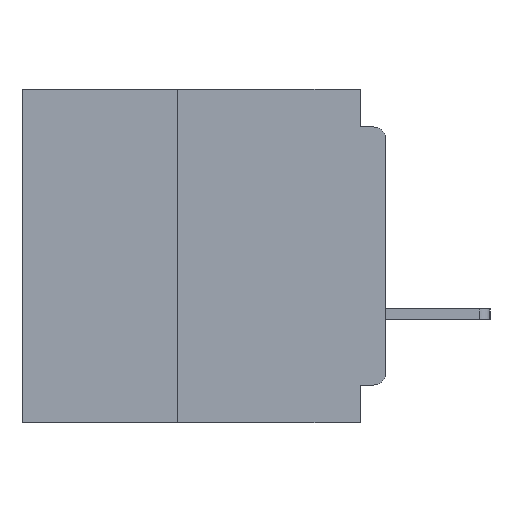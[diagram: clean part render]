
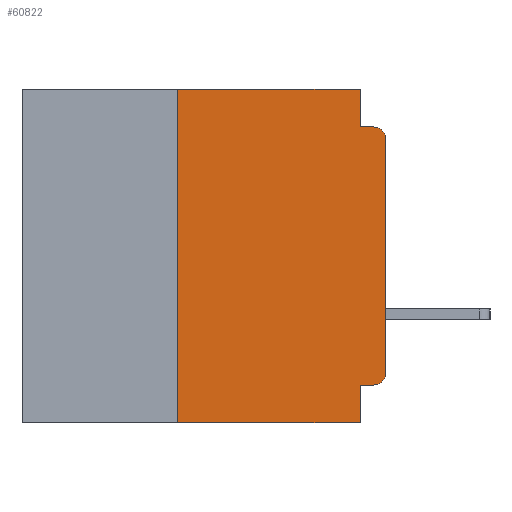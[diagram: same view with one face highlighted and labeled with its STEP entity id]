
A CAD part, left-side view. The second image highlights one B-rep face of the part: STEP entity #60822.
In plain terms, the highlighted planar face has unit normal (-1, 0, 0).
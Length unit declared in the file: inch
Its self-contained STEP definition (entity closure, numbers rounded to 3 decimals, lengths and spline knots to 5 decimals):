
#879 = VECTOR ( 'NONE', #21211, 39.37008 ) ;
#1084 = LINE ( 'NONE', #3844, #49012 ) ;
#2308 = LINE ( 'NONE', #2730, #51685 ) ;
#2730 = CARTESIAN_POINT ( 'NONE',  ( 0., 0.437, 0. ) ) ;
#3196 = LINE ( 'NONE', #24587, #39939 ) ;
#3844 = CARTESIAN_POINT ( 'NONE',  ( 0., 0.031, -0.4 ) ) ;
#6671 = LINE ( 'NONE', #43525, #29167 ) ;
#6939 = CARTESIAN_POINT ( 'NONE',  ( 0., 0.25, 0. ) ) ;
#6957 = AXIS2_PLACEMENT_3D ( 'NONE', #60217, #41269, #12670 ) ;
#7172 = CARTESIAN_POINT ( 'NONE',  ( 0., 0.015, -0.045 ) ) ;
#7630 = PLANE ( 'NONE',  #6957 ) ;
#7740 = AXIS2_PLACEMENT_3D ( 'NONE', #54653, #26186, #59476 ) ;
#8360 = EDGE_CURVE ( 'NONE', #43279, #45960, #3196, .T. ) ;
#8564 = EDGE_CURVE ( 'NONE', #43279, #43929, #13726, .T. ) ;
#9589 = ORIENTED_EDGE ( 'NONE', *, *, #12845, .F. ) ;
#9753 = DIRECTION ( 'NONE',  ( 0., 1., 0. ) ) ;
#10267 = VECTOR ( 'NONE', #9753, 39.37008 ) ;
#11570 = CARTESIAN_POINT ( 'NONE',  ( 0., 0.437, -0.4 ) ) ;
#12670 = DIRECTION ( 'NONE',  ( 0., 0., -1. ) ) ;
#12845 = EDGE_CURVE ( 'NONE', #45960, #54030, #2308, .T. ) ;
#12960 = CARTESIAN_POINT ( 'NONE',  ( 0., 0.015, -0.355 ) ) ;
#13506 = EDGE_LOOP ( 'NONE', ( #56353, #36671, #37065, #57245, #9589, #48630, #24536, #41566, #30895, #26629 ) ) ;
#13726 = LINE ( 'NONE', #11570, #879 ) ;
#13753 = LINE ( 'NONE', #45298, #25012 ) ;
#14401 = CARTESIAN_POINT ( 'NONE',  ( 0., 0., -0.355 ) ) ;
#14575 = CARTESIAN_POINT ( 'NONE',  ( 0., 0.25, -0.4 ) ) ;
#14997 = VERTEX_POINT ( 'NONE', #12960 ) ;
#15764 = VERTEX_POINT ( 'NONE', #42906 ) ;
#21211 = DIRECTION ( 'NONE',  ( 0., -1., 0. ) ) ;
#21439 = VERTEX_POINT ( 'NONE', #60496 ) ;
#22105 = CARTESIAN_POINT ( 'NONE',  ( 0., 0.031, 0. ) ) ;
#22118 = DIRECTION ( 'NONE',  ( 0., -1., 0. ) ) ;
#24536 = ORIENTED_EDGE ( 'NONE', *, *, #8564, .T. ) ;
#24587 = CARTESIAN_POINT ( 'NONE',  ( 0., 0.25, -0.4 ) ) ;
#25012 = VECTOR ( 'NONE', #26354, 39.37008 ) ;
#25108 = EDGE_CURVE ( 'NONE', #54030, #30699, #26549, .T. ) ;
#25467 = DIRECTION ( 'NONE',  ( -1., 0., 0. ) ) ;
#26186 = DIRECTION ( 'NONE',  ( -1., 0., 0. ) ) ;
#26354 = DIRECTION ( 'NONE',  ( 0., 0., 1. ) ) ;
#26549 = LINE ( 'NONE', #22105, #28025 ) ;
#26629 = ORIENTED_EDGE ( 'NONE', *, *, #35630, .T. ) ;
#28025 = VECTOR ( 'NONE', #55391, 39.37008 ) ;
#29167 = VECTOR ( 'NONE', #48309, 39.37008 ) ;
#30063 = CARTESIAN_POINT ( 'NONE',  ( 0., 0.031, -0.045 ) ) ;
#30699 = VERTEX_POINT ( 'NONE', #30063 ) ;
#30895 = ORIENTED_EDGE ( 'NONE', *, *, #39320, .F. ) ;
#32015 = EDGE_CURVE ( 'NONE', #15764, #21439, #13753, .T. ) ;
#32635 = VERTEX_POINT ( 'NONE', #7172 ) ;
#33608 = CARTESIAN_POINT ( 'NONE',  ( 0., 0.031, 0. ) ) ;
#35630 = EDGE_CURVE ( 'NONE', #14997, #15764, #51741, .T. ) ;
#36656 = AXIS2_PLACEMENT_3D ( 'NONE', #53970, #25467, #58790 ) ;
#36671 = ORIENTED_EDGE ( 'NONE', *, *, #61506, .T. ) ;
#37065 = ORIENTED_EDGE ( 'NONE', *, *, #57135, .F. ) ;
#37228 = LINE ( 'NONE', #14401, #10267 ) ;
#38965 = DIRECTION ( 'NONE',  ( 0., 0., 1. ) ) ;
#39320 = EDGE_CURVE ( 'NONE', #14997, #51120, #37228, .T. ) ;
#39939 = VECTOR ( 'NONE', #38965, 39.37008 ) ;
#40034 = CIRCLE ( 'NONE', #36656, 0.015 ) ;
#41269 = DIRECTION ( 'NONE',  ( 1., 0., 0. ) ) ;
#41566 = ORIENTED_EDGE ( 'NONE', *, *, #60302, .F. ) ;
#42141 = DIRECTION ( 'NONE',  ( 0., 0., -1. ) ) ;
#42906 = CARTESIAN_POINT ( 'NONE',  ( 0., 0., -0.34 ) ) ;
#43279 = VERTEX_POINT ( 'NONE', #14575 ) ;
#43525 = CARTESIAN_POINT ( 'NONE',  ( 0., 0., -0.045 ) ) ;
#43929 = VERTEX_POINT ( 'NONE', #48074 ) ;
#45298 = CARTESIAN_POINT ( 'NONE',  ( 0., 0., 0. ) ) ;
#45960 = VERTEX_POINT ( 'NONE', #6939 ) ;
#46855 = CARTESIAN_POINT ( 'NONE',  ( 0., 0.031, -0.355 ) ) ;
#48074 = CARTESIAN_POINT ( 'NONE',  ( 0., 0.031, -0.4 ) ) ;
#48309 = DIRECTION ( 'NONE',  ( 0., -1., 0. ) ) ;
#48630 = ORIENTED_EDGE ( 'NONE', *, *, #8360, .F. ) ;
#49012 = VECTOR ( 'NONE', #42141, 39.37008 ) ;
#51120 = VERTEX_POINT ( 'NONE', #46855 ) ;
#51685 = VECTOR ( 'NONE', #22118, 39.37008 ) ;
#51741 = CIRCLE ( 'NONE', #7740, 0.015 ) ;
#53970 = CARTESIAN_POINT ( 'NONE',  ( 0., 0.015, -0.06 ) ) ;
#54030 = VERTEX_POINT ( 'NONE', #33608 ) ;
#54653 = CARTESIAN_POINT ( 'NONE',  ( 0., 0.015, -0.34 ) ) ;
#55391 = DIRECTION ( 'NONE',  ( 0., 0., -1. ) ) ;
#55626 = FACE_OUTER_BOUND ( 'NONE', #13506, .T. ) ;
#56353 = ORIENTED_EDGE ( 'NONE', *, *, #32015, .T. ) ;
#57135 = EDGE_CURVE ( 'NONE', #30699, #32635, #6671, .T. ) ;
#57245 = ORIENTED_EDGE ( 'NONE', *, *, #25108, .F. ) ;
#58790 = DIRECTION ( 'NONE',  ( 0., 0., -1. ) ) ;
#59476 = DIRECTION ( 'NONE',  ( 0., 0., -1. ) ) ;
#60217 = CARTESIAN_POINT ( 'NONE',  ( 0., 0.437, 0. ) ) ;
#60302 = EDGE_CURVE ( 'NONE', #51120, #43929, #1084, .T. ) ;
#60496 = CARTESIAN_POINT ( 'NONE',  ( 0., 0., -0.06 ) ) ;
#60822 = ADVANCED_FACE ( 'NONE', ( #55626 ), #7630, .F. ) ;
#61506 = EDGE_CURVE ( 'NONE', #21439, #32635, #40034, .T. ) ;
